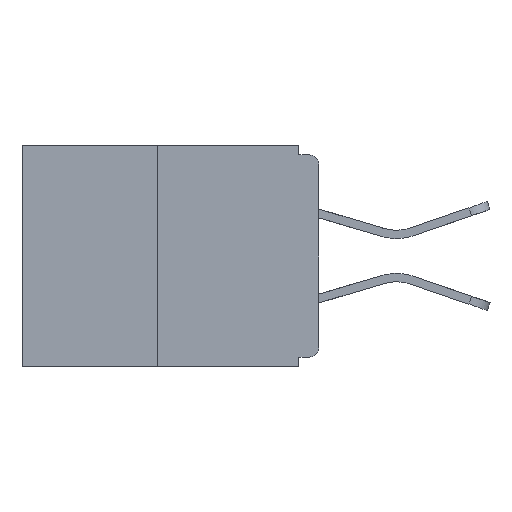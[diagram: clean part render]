
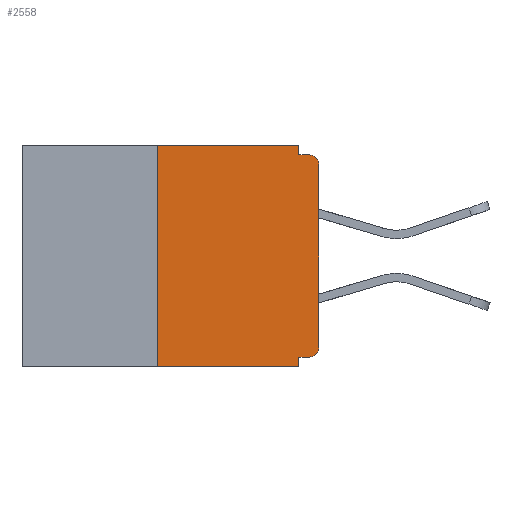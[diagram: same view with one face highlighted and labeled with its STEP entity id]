
A CAD part, left-side view. The second image highlights one B-rep face of the part: STEP entity #2558.
In plain terms, the highlighted planar face has unit normal (-1, 0, 0).
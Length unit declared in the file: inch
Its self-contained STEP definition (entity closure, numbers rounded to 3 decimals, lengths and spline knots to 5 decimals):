
#189 = DIRECTION ( 'NONE',  ( 1., 0., 0. ) ) ;
#252 = DIRECTION ( 'NONE',  ( 0., 0., -1. ) ) ;
#341 = ORIENTED_EDGE ( 'NONE', *, *, #9036, .T. ) ;
#442 = CARTESIAN_POINT ( 'NONE',  ( 0., 0.015, -0.313 ) ) ;
#473 = VERTEX_POINT ( 'NONE', #543 ) ;
#543 = CARTESIAN_POINT ( 'NONE',  ( 0., 0.031, -0.343 ) ) ;
#555 = CARTESIAN_POINT ( 'NONE',  ( 0., 0.015, -0.328 ) ) ;
#614 = VERTEX_POINT ( 'NONE', #5892 ) ;
#1179 = CIRCLE ( 'NONE', #11239, 0.015 ) ;
#1325 = VECTOR ( 'NONE', #5294, 39.37008 ) ;
#1561 = DIRECTION ( 'NONE',  ( -1., 0., 0. ) ) ;
#2056 = EDGE_CURVE ( 'NONE', #2727, #473, #4925, .T. ) ;
#2440 = ORIENTED_EDGE ( 'NONE', *, *, #15485, .T. ) ;
#2491 = ORIENTED_EDGE ( 'NONE', *, *, #13254, .F. ) ;
#2558 = ADVANCED_FACE ( 'NONE', ( #6596 ), #12428, .F. ) ;
#2564 = ORIENTED_EDGE ( 'NONE', *, *, #14666, .T. ) ;
#2727 = VERTEX_POINT ( 'NONE', #7903 ) ;
#2731 = DIRECTION ( 'NONE',  ( 0., 0., -1. ) ) ;
#3266 = VERTEX_POINT ( 'NONE', #17085 ) ;
#3404 = DIRECTION ( 'NONE',  ( 0., 1., 0. ) ) ;
#3898 = ORIENTED_EDGE ( 'NONE', *, *, #16168, .F. ) ;
#3916 = CARTESIAN_POINT ( 'NONE',  ( 0., 0.25, 0. ) ) ;
#4077 = EDGE_CURVE ( 'NONE', #14806, #12006, #8002, .T. ) ;
#4182 = DIRECTION ( 'NONE',  ( 0., -1., 0. ) ) ;
#4374 = LINE ( 'NONE', #3916, #16238 ) ;
#4607 = VERTEX_POINT ( 'NONE', #12985 ) ;
#4815 = CARTESIAN_POINT ( 'NONE',  ( 0., 0., -0.328 ) ) ;
#4925 = LINE ( 'NONE', #14873, #1325 ) ;
#5278 = CARTESIAN_POINT ( 'NONE',  ( 0., 0., 0. ) ) ;
#5294 = DIRECTION ( 'NONE',  ( 0., 0., -1. ) ) ;
#5321 = LINE ( 'NONE', #4815, #8504 ) ;
#5499 = ORIENTED_EDGE ( 'NONE', *, *, #4077, .T. ) ;
#5892 = CARTESIAN_POINT ( 'NONE',  ( 0., 0.25, -0.343 ) ) ;
#5895 = VERTEX_POINT ( 'NONE', #15815 ) ;
#5904 = AXIS2_PLACEMENT_3D ( 'NONE', #442, #7294, #12629 ) ;
#5968 = ORIENTED_EDGE ( 'NONE', *, *, #2056, .F. ) ;
#6255 = LINE ( 'NONE', #5278, #17470 ) ;
#6454 = LINE ( 'NONE', #7115, #6661 ) ;
#6596 = FACE_OUTER_BOUND ( 'NONE', #7699, .T. ) ;
#6661 = VECTOR ( 'NONE', #12572, 39.37008 ) ;
#6980 = ORIENTED_EDGE ( 'NONE', *, *, #8026, .F. ) ;
#7115 = CARTESIAN_POINT ( 'NONE',  ( 0., 0.46, 0. ) ) ;
#7294 = DIRECTION ( 'NONE',  ( -1., 0., 0. ) ) ;
#7603 = AXIS2_PLACEMENT_3D ( 'NONE', #8287, #189, #252 ) ;
#7699 = EDGE_LOOP ( 'NONE', ( #3898, #2491, #341, #5968, #13827, #5499, #2440, #2564, #10918, #6980 ) ) ;
#7903 = CARTESIAN_POINT ( 'NONE',  ( 0., 0.031, -0.328 ) ) ;
#8002 = CIRCLE ( 'NONE', #5904, 0.015 ) ;
#8026 = EDGE_CURVE ( 'NONE', #3266, #15424, #10402, .T. ) ;
#8137 = DIRECTION ( 'NONE',  ( 0., 0., -1. ) ) ;
#8287 = CARTESIAN_POINT ( 'NONE',  ( 0., 0.46, 0. ) ) ;
#8504 = VECTOR ( 'NONE', #3404, 39.37008 ) ;
#8515 = DIRECTION ( 'NONE',  ( 0., -1., 0. ) ) ;
#9036 = EDGE_CURVE ( 'NONE', #614, #473, #12398, .T. ) ;
#9538 = LINE ( 'NONE', #15015, #11871 ) ;
#9542 = DIRECTION ( 'NONE',  ( 0., 0., 1. ) ) ;
#10402 = LINE ( 'NONE', #13759, #14629 ) ;
#10609 = DIRECTION ( 'NONE',  ( 0., 0., 1. ) ) ;
#10918 = ORIENTED_EDGE ( 'NONE', *, *, #11582, .F. ) ;
#10947 = EDGE_CURVE ( 'NONE', #14806, #2727, #5321, .T. ) ;
#11012 = VERTEX_POINT ( 'NONE', #15561 ) ;
#11227 = CARTESIAN_POINT ( 'NONE',  ( 0., 0.46, -0.343 ) ) ;
#11239 = AXIS2_PLACEMENT_3D ( 'NONE', #13525, #1561, #8137 ) ;
#11351 = CARTESIAN_POINT ( 'NONE',  ( 0., 0., -0.313 ) ) ;
#11582 = EDGE_CURVE ( 'NONE', #15424, #4607, #9538, .T. ) ;
#11795 = CARTESIAN_POINT ( 'NONE',  ( 0., 0.031, -0.015 ) ) ;
#11871 = VECTOR ( 'NONE', #4182, 39.37008 ) ;
#12006 = VERTEX_POINT ( 'NONE', #11351 ) ;
#12398 = LINE ( 'NONE', #11227, #15344 ) ;
#12428 = PLANE ( 'NONE',  #7603 ) ;
#12572 = DIRECTION ( 'NONE',  ( 0., -1., 0. ) ) ;
#12629 = DIRECTION ( 'NONE',  ( 0., 0., -1. ) ) ;
#12985 = CARTESIAN_POINT ( 'NONE',  ( 0., 0.015, -0.015 ) ) ;
#13254 = EDGE_CURVE ( 'NONE', #614, #5895, #4374, .T. ) ;
#13525 = CARTESIAN_POINT ( 'NONE',  ( 0., 0.015, -0.03 ) ) ;
#13759 = CARTESIAN_POINT ( 'NONE',  ( 0., 0.031, 0. ) ) ;
#13827 = ORIENTED_EDGE ( 'NONE', *, *, #10947, .F. ) ;
#14629 = VECTOR ( 'NONE', #2731, 39.37008 ) ;
#14666 = EDGE_CURVE ( 'NONE', #11012, #4607, #1179, .T. ) ;
#14806 = VERTEX_POINT ( 'NONE', #555 ) ;
#14873 = CARTESIAN_POINT ( 'NONE',  ( 0., 0.031, -0.343 ) ) ;
#15015 = CARTESIAN_POINT ( 'NONE',  ( 0., 0., -0.015 ) ) ;
#15344 = VECTOR ( 'NONE', #8515, 39.37008 ) ;
#15424 = VERTEX_POINT ( 'NONE', #11795 ) ;
#15485 = EDGE_CURVE ( 'NONE', #12006, #11012, #6255, .T. ) ;
#15561 = CARTESIAN_POINT ( 'NONE',  ( 0., 0., -0.03 ) ) ;
#15815 = CARTESIAN_POINT ( 'NONE',  ( 0., 0.25, 0. ) ) ;
#16168 = EDGE_CURVE ( 'NONE', #5895, #3266, #6454, .T. ) ;
#16238 = VECTOR ( 'NONE', #10609, 39.37008 ) ;
#17085 = CARTESIAN_POINT ( 'NONE',  ( 0., 0.031, 0. ) ) ;
#17470 = VECTOR ( 'NONE', #9542, 39.37008 ) ;
